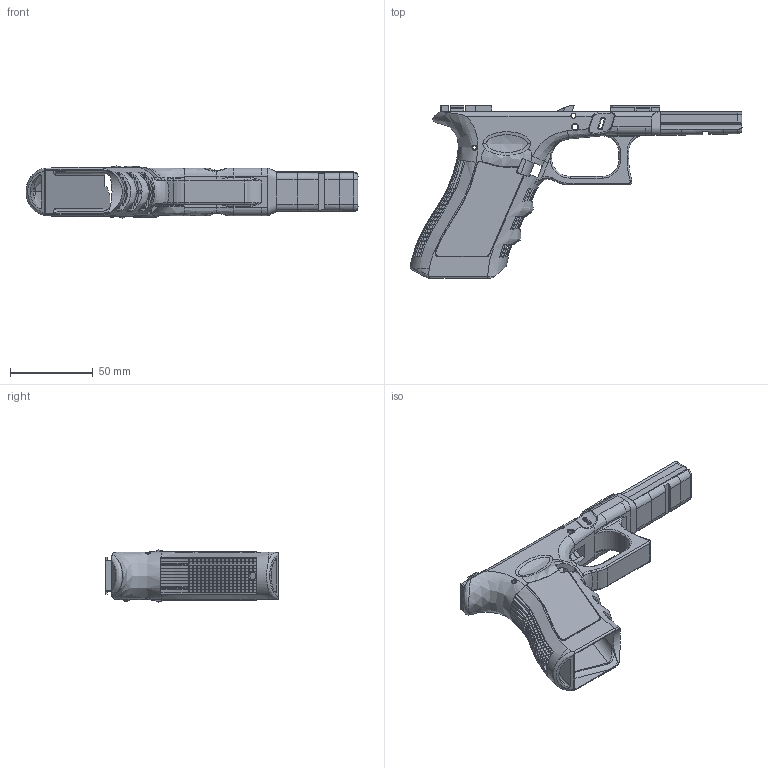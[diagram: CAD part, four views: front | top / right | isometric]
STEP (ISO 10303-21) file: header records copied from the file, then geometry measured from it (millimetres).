
FILE_DESCRIPTION (( 'STEP AP214' ), '1' );
FILE_NAME ('Glock-Gen3-Ramp.STEP', '2018-08-01T19:09:19', ( '' ), ( '' ), 'SwSTEP 2.0', 'SolidWorks 2015', '' );
FILE_SCHEMA (( 'AUTOMOTIVE_DESIGN' ));
Length unit declared in the file: millimetre
Products named in the file (1): Glock-Gen3-Ramp
Bounding box: 201.04 x 104.61 x 31.52 mm (x, y, z)
Volume: 80803.9 mm3; surface area: 51227 mm2
Topology: 1 solids, 1 shells, 1895 faces, 4568 edges, 2662 vertices
Faces by surface type: plane 1105, bspline 563, cylinder 168, torus 43, sphere 10, cone 6
Entity records: 115174 total; most frequent: CARTESIAN_POINT 77025, ORIENTED_EDGE 9112, DIRECTION 5284, EDGE_CURVE 4556, VERTEX_POINT 2659, B_SPLINE_CURVE_WITH_KNOTS 2268, EDGE_LOOP 1921, ADVANCED_FACE 1895
